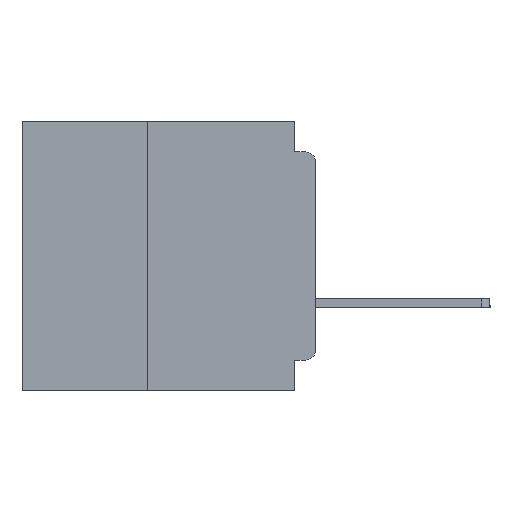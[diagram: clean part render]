
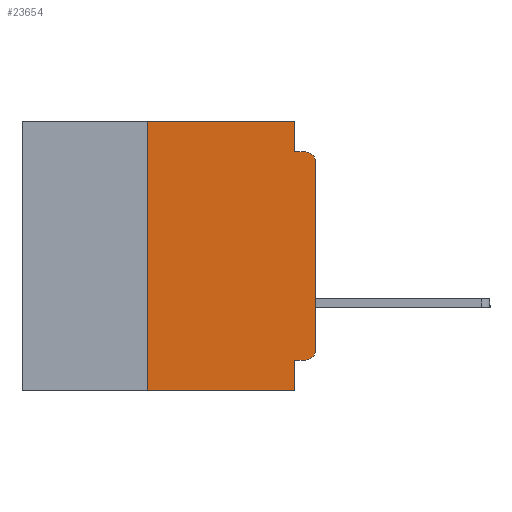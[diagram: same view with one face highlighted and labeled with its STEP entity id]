
A CAD part, left-side view. The second image highlights one B-rep face of the part: STEP entity #23654.
In plain terms, the highlighted planar face has unit normal (-1, 0, 0).
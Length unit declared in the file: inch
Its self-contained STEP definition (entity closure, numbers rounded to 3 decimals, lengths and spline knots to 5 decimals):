
#95 = CARTESIAN_POINT ( 'NONE',  ( 0., 0.015, -0.06 ) ) ;
#257 = VECTOR ( 'NONE', #29255, 39.37008 ) ;
#288 = CARTESIAN_POINT ( 'NONE',  ( 0., 0.015, -0.045 ) ) ;
#339 = VERTEX_POINT ( 'NONE', #45044 ) ;
#532 = CARTESIAN_POINT ( 'NONE',  ( 0., 0., -0.045 ) ) ;
#1058 = VECTOR ( 'NONE', #36686, 39.37008 ) ;
#1660 = CARTESIAN_POINT ( 'NONE',  ( 0., 0., 0. ) ) ;
#2294 = CARTESIAN_POINT ( 'NONE',  ( 0., 0.031, -0.4 ) ) ;
#2735 = VECTOR ( 'NONE', #22209, 39.37008 ) ;
#3983 = DIRECTION ( 'NONE',  ( 0., 0., -1. ) ) ;
#4004 = AXIS2_PLACEMENT_3D ( 'NONE', #95, #27016, #3983 ) ;
#4266 = VERTEX_POINT ( 'NONE', #9142 ) ;
#6472 = ORIENTED_EDGE ( 'NONE', *, *, #36880, .F. ) ;
#7635 = ORIENTED_EDGE ( 'NONE', *, *, #28637, .T. ) ;
#8319 = CARTESIAN_POINT ( 'NONE',  ( 0., 0.437, 0. ) ) ;
#8497 = CARTESIAN_POINT ( 'NONE',  ( 0., 0.015, -0.355 ) ) ;
#8665 = EDGE_CURVE ( 'NONE', #45286, #43690, #12923, .T. ) ;
#9128 = EDGE_CURVE ( 'NONE', #339, #43690, #29817, .T. ) ;
#9142 = CARTESIAN_POINT ( 'NONE',  ( 0., 0., -0.06 ) ) ;
#9482 = VECTOR ( 'NONE', #39145, 39.37008 ) ;
#10356 = VERTEX_POINT ( 'NONE', #28958 ) ;
#10380 = CARTESIAN_POINT ( 'NONE',  ( 0., 0., -0.355 ) ) ;
#10603 = CARTESIAN_POINT ( 'NONE',  ( 0., 0.437, -0.4 ) ) ;
#11112 = CARTESIAN_POINT ( 'NONE',  ( 0., 0.031, 0. ) ) ;
#11325 = LINE ( 'NONE', #25018, #1058 ) ;
#11411 = CIRCLE ( 'NONE', #40104, 0.015 ) ;
#12024 = ORIENTED_EDGE ( 'NONE', *, *, #30373, .F. ) ;
#12923 = LINE ( 'NONE', #10603, #2735 ) ;
#13642 = EDGE_LOOP ( 'NONE', ( #46428, #7635, #27999, #6472, #19398, #15654, #32147, #33487, #12024, #41466 ) ) ;
#13755 = LINE ( 'NONE', #45473, #44539 ) ;
#15380 = CARTESIAN_POINT ( 'NONE',  ( 0., 0.015, -0.34 ) ) ;
#15654 = ORIENTED_EDGE ( 'NONE', *, *, #43368, .F. ) ;
#15906 = CIRCLE ( 'NONE', #4004, 0.015 ) ;
#17148 = VERTEX_POINT ( 'NONE', #43919 ) ;
#18190 = LINE ( 'NONE', #10380, #30906 ) ;
#18282 = EDGE_CURVE ( 'NONE', #17148, #36006, #40242, .T. ) ;
#18735 = VERTEX_POINT ( 'NONE', #11112 ) ;
#19296 = DIRECTION ( 'NONE',  ( 0., 0., -1. ) ) ;
#19398 = ORIENTED_EDGE ( 'NONE', *, *, #47621, .F. ) ;
#19879 = DIRECTION ( 'NONE',  ( 1., 0., 0. ) ) ;
#21637 = CARTESIAN_POINT ( 'NONE',  ( 0., 0.25, 0. ) ) ;
#22209 = DIRECTION ( 'NONE',  ( 0., -1., 0. ) ) ;
#23654 = ADVANCED_FACE ( 'NONE', ( #39683 ), #46642, .F. ) ;
#25018 = CARTESIAN_POINT ( 'NONE',  ( 0., 0.031, 0. ) ) ;
#26179 = CARTESIAN_POINT ( 'NONE',  ( 0., 0.437, 0. ) ) ;
#27016 = DIRECTION ( 'NONE',  ( -1., 0., 0. ) ) ;
#27999 = ORIENTED_EDGE ( 'NONE', *, *, #18282, .F. ) ;
#28024 = AXIS2_PLACEMENT_3D ( 'NONE', #8319, #19879, #46797 ) ;
#28637 = EDGE_CURVE ( 'NONE', #4266, #36006, #15906, .T. ) ;
#28958 = CARTESIAN_POINT ( 'NONE',  ( 0., 0., -0.34 ) ) ;
#29255 = DIRECTION ( 'NONE',  ( 0., 0., -1. ) ) ;
#29817 = LINE ( 'NONE', #2294, #257 ) ;
#30373 = EDGE_CURVE ( 'NONE', #35040, #339, #18190, .T. ) ;
#30906 = VECTOR ( 'NONE', #37351, 39.37008 ) ;
#31203 = VECTOR ( 'NONE', #32518, 39.37008 ) ;
#31984 = CARTESIAN_POINT ( 'NONE',  ( 0., 0.031, -0.4 ) ) ;
#32147 = ORIENTED_EDGE ( 'NONE', *, *, #8665, .T. ) ;
#32518 = DIRECTION ( 'NONE',  ( 0., 0., 1. ) ) ;
#33487 = ORIENTED_EDGE ( 'NONE', *, *, #9128, .F. ) ;
#35040 = VERTEX_POINT ( 'NONE', #8497 ) ;
#35958 = CARTESIAN_POINT ( 'NONE',  ( 0., 0.25, -0.4 ) ) ;
#35969 = EDGE_CURVE ( 'NONE', #35040, #10356, #11411, .T. ) ;
#36006 = VERTEX_POINT ( 'NONE', #288 ) ;
#36686 = DIRECTION ( 'NONE',  ( 0., 0., -1. ) ) ;
#36880 = EDGE_CURVE ( 'NONE', #18735, #17148, #11325, .T. ) ;
#37351 = DIRECTION ( 'NONE',  ( 0., 1., 0. ) ) ;
#38137 = EDGE_CURVE ( 'NONE', #10356, #4266, #41459, .T. ) ;
#39145 = DIRECTION ( 'NONE',  ( 0., -1., 0. ) ) ;
#39683 = FACE_OUTER_BOUND ( 'NONE', #13642, .T. ) ;
#40104 = AXIS2_PLACEMENT_3D ( 'NONE', #15380, #42406, #19296 ) ;
#40242 = LINE ( 'NONE', #532, #9482 ) ;
#41459 = LINE ( 'NONE', #1660, #31203 ) ;
#41466 = ORIENTED_EDGE ( 'NONE', *, *, #35969, .T. ) ;
#41541 = DIRECTION ( 'NONE',  ( 0., -1., 0. ) ) ;
#42406 = DIRECTION ( 'NONE',  ( -1., 0., 0. ) ) ;
#43368 = EDGE_CURVE ( 'NONE', #45286, #46703, #13755, .T. ) ;
#43690 = VERTEX_POINT ( 'NONE', #31984 ) ;
#43868 = LINE ( 'NONE', #26179, #45094 ) ;
#43919 = CARTESIAN_POINT ( 'NONE',  ( 0., 0.031, -0.045 ) ) ;
#44539 = VECTOR ( 'NONE', #45309, 39.37008 ) ;
#45044 = CARTESIAN_POINT ( 'NONE',  ( 0., 0.031, -0.355 ) ) ;
#45094 = VECTOR ( 'NONE', #41541, 39.37008 ) ;
#45286 = VERTEX_POINT ( 'NONE', #35958 ) ;
#45309 = DIRECTION ( 'NONE',  ( 0., 0., 1. ) ) ;
#45473 = CARTESIAN_POINT ( 'NONE',  ( 0., 0.25, -0.4 ) ) ;
#46428 = ORIENTED_EDGE ( 'NONE', *, *, #38137, .T. ) ;
#46642 = PLANE ( 'NONE',  #28024 ) ;
#46703 = VERTEX_POINT ( 'NONE', #21637 ) ;
#46797 = DIRECTION ( 'NONE',  ( 0., 0., -1. ) ) ;
#47621 = EDGE_CURVE ( 'NONE', #46703, #18735, #43868, .T. ) ;
